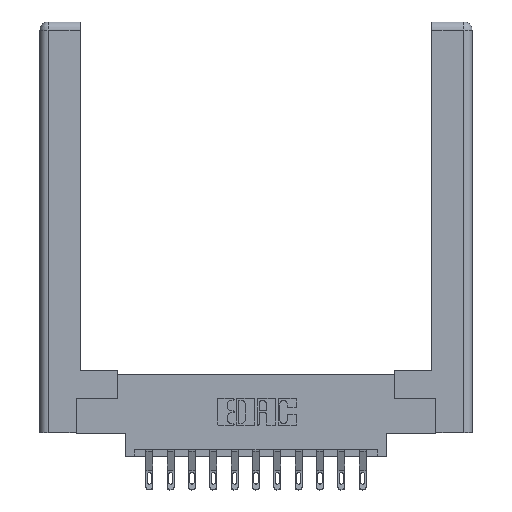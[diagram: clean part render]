
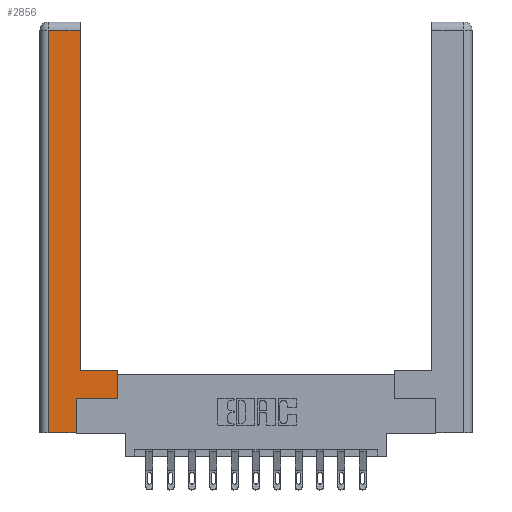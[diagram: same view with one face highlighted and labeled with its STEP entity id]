
A CAD part, top view. The second image highlights one B-rep face of the part: STEP entity #2856.
In plain terms, the highlighted planar face has unit normal (0, 0, 1).
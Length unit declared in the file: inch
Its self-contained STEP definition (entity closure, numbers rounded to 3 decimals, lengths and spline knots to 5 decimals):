
#99 = VECTOR ( 'NONE', #13251, 39.37008 ) ;
#146 = ORIENTED_EDGE ( 'NONE', *, *, #10696, .T. ) ;
#497 = AXIS2_PLACEMENT_3D ( 'NONE', #14428, #11974, #4765 ) ;
#501 = VECTOR ( 'NONE', #11133, 39.37008 ) ;
#973 = CARTESIAN_POINT ( 'NONE',  ( 0.565, 0.245, 0. ) ) ;
#1153 = VERTEX_POINT ( 'NONE', #9832 ) ;
#1425 = ORIENTED_EDGE ( 'NONE', *, *, #6866, .T. ) ;
#1518 = LINE ( 'NONE', #12012, #7572 ) ;
#1819 = VERTEX_POINT ( 'NONE', #12109 ) ;
#1883 = DIRECTION ( 'NONE',  ( -1., 0., 0. ) ) ;
#2333 = LINE ( 'NONE', #6259, #8394 ) ;
#2438 = EDGE_CURVE ( 'NONE', #7666, #4854, #13156, .T. ) ;
#2655 = DIRECTION ( 'NONE',  ( 1., 0., 0. ) ) ;
#2856 = ADVANCED_FACE ( 'NONE', ( #5205 ), #10754, .F. ) ;
#2937 = LINE ( 'NONE', #9565, #99 ) ;
#3090 = VERTEX_POINT ( 'NONE', #4190 ) ;
#3124 = VERTEX_POINT ( 'NONE', #11335 ) ;
#3160 = EDGE_LOOP ( 'NONE', ( #1425, #14482, #8389, #9537, #4494, #14692, #9117, #146 ) ) ;
#3526 = EDGE_CURVE ( 'NONE', #3124, #3090, #2937, .T. ) ;
#3913 = VECTOR ( 'NONE', #9080, 39.37008 ) ;
#4002 = CARTESIAN_POINT ( 'NONE',  ( 0.265, 0., 0. ) ) ;
#4190 = CARTESIAN_POINT ( 'NONE',  ( 0.265, 0.245, 0. ) ) ;
#4268 = CARTESIAN_POINT ( 'NONE',  ( 0.565, 0.45, 0. ) ) ;
#4412 = LINE ( 'NONE', #9572, #9099 ) ;
#4453 = CARTESIAN_POINT ( 'NONE',  ( 0.0615, 2.94, 0. ) ) ;
#4494 = ORIENTED_EDGE ( 'NONE', *, *, #3526, .T. ) ;
#4765 = DIRECTION ( 'NONE',  ( -1., 0., 0. ) ) ;
#4828 = EDGE_CURVE ( 'NONE', #1153, #3124, #12828, .T. ) ;
#4854 = VERTEX_POINT ( 'NONE', #6408 ) ;
#5012 = DIRECTION ( 'NONE',  ( 0., -1., 0. ) ) ;
#5095 = VECTOR ( 'NONE', #2655, 39.37008 ) ;
#5205 = FACE_OUTER_BOUND ( 'NONE', #3160, .T. ) ;
#6259 = CARTESIAN_POINT ( 'NONE',  ( 0.0615, 0., 0. ) ) ;
#6408 = CARTESIAN_POINT ( 'NONE',  ( 0.565, 0.45, 0. ) ) ;
#6866 = EDGE_CURVE ( 'NONE', #12492, #9656, #14331, .T. ) ;
#7430 = DIRECTION ( 'NONE',  ( -1., 0., 0. ) ) ;
#7572 = VECTOR ( 'NONE', #7430, 39.37008 ) ;
#7603 = DIRECTION ( 'NONE',  ( 1., 0., 0. ) ) ;
#7637 = CARTESIAN_POINT ( 'NONE',  ( 0.295, 2.94, 0. ) ) ;
#7666 = VERTEX_POINT ( 'NONE', #973 ) ;
#8389 = ORIENTED_EDGE ( 'NONE', *, *, #13978, .T. ) ;
#8394 = VECTOR ( 'NONE', #5012, 39.37008 ) ;
#9080 = DIRECTION ( 'NONE',  ( 0., 1., 0. ) ) ;
#9099 = VECTOR ( 'NONE', #7603, 39.37008 ) ;
#9117 = ORIENTED_EDGE ( 'NONE', *, *, #2438, .T. ) ;
#9537 = ORIENTED_EDGE ( 'NONE', *, *, #4828, .T. ) ;
#9565 = CARTESIAN_POINT ( 'NONE',  ( 0.265, 0.245, 0. ) ) ;
#9572 = CARTESIAN_POINT ( 'NONE',  ( 0.565, 0.245, 0. ) ) ;
#9656 = VERTEX_POINT ( 'NONE', #7637 ) ;
#9832 = CARTESIAN_POINT ( 'NONE',  ( 0.0615, 0., 0. ) ) ;
#10513 = EDGE_CURVE ( 'NONE', #9656, #1819, #14010, .T. ) ;
#10696 = EDGE_CURVE ( 'NONE', #4854, #12492, #1518, .T. ) ;
#10754 = PLANE ( 'NONE',  #497 ) ;
#11133 = DIRECTION ( 'NONE',  ( 0., 1., 0. ) ) ;
#11335 = CARTESIAN_POINT ( 'NONE',  ( 0.265, 0., 0. ) ) ;
#11974 = DIRECTION ( 'NONE',  ( 0., 0., -1. ) ) ;
#12012 = CARTESIAN_POINT ( 'NONE',  ( 0.295, 0.45, 0. ) ) ;
#12109 = CARTESIAN_POINT ( 'NONE',  ( 0.0615, 2.94, 0. ) ) ;
#12472 = VECTOR ( 'NONE', #1883, 39.37008 ) ;
#12492 = VERTEX_POINT ( 'NONE', #13132 ) ;
#12828 = LINE ( 'NONE', #4002, #5095 ) ;
#13132 = CARTESIAN_POINT ( 'NONE',  ( 0.295, 0.45, 0. ) ) ;
#13156 = LINE ( 'NONE', #4268, #3913 ) ;
#13251 = DIRECTION ( 'NONE',  ( 0., 1., 0. ) ) ;
#13978 = EDGE_CURVE ( 'NONE', #1819, #1153, #2333, .T. ) ;
#14010 = LINE ( 'NONE', #4453, #12472 ) ;
#14331 = LINE ( 'NONE', #14854, #501 ) ;
#14428 = CARTESIAN_POINT ( 'NONE',  ( 0., 0., 0. ) ) ;
#14482 = ORIENTED_EDGE ( 'NONE', *, *, #10513, .T. ) ;
#14692 = ORIENTED_EDGE ( 'NONE', *, *, #15261, .T. ) ;
#14854 = CARTESIAN_POINT ( 'NONE',  ( 0.295, 3., 0. ) ) ;
#15261 = EDGE_CURVE ( 'NONE', #3090, #7666, #4412, .T. ) ;
